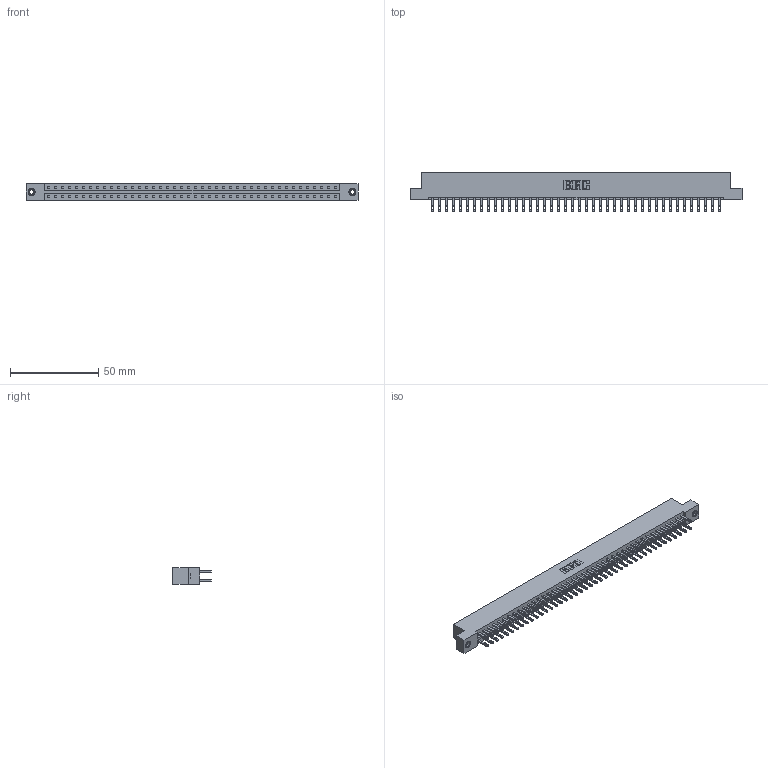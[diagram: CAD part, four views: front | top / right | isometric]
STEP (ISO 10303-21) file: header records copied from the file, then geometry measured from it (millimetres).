
FILE_DESCRIPTION (( 'STEP AP203' ), '1' );
FILE_NAME ('333-084-500-207.STEP', '2018-08-05T03:57:02', ( '' ), ( '' ), 'SwSTEP 2.0', 'SolidWorks 2016', '' );
FILE_SCHEMA (( 'CONFIG_CONTROL_DESIGN' ));
Length unit declared in the file: inch
Products named in the file (4): 333 Part_Flush - .156 Dia - TI; 345-292-001_345-293-100; 345-250-001_345-250-005-103; 333-084-500-207
Assembly tree (87 placements, depth 2):
  333-084-500-207
    333 Part_Flush - .156 Dia - TI
    345-292-001_345-293-100  x84
    345-250-001_345-250-005-103  x2
Bounding box: 187.96 x 21.85 x 9.4 mm (x, y, z)
Volume: 19432.8 mm3; surface area: 23932.9 mm2
Topology: 87 solids, 87 shells, 4206 faces, 12795 edges, 8522 vertices
Faces by surface type: plane 2622, cylinder 1568, cone 12, torus 4
Entity records: 28136 total; most frequent: CARTESIAN_POINT 4645, ORIENTED_EDGE 4574, DIRECTION 4001, EDGE_CURVE 2287, LINE 2135, VECTOR 2135, VERTEX_POINT 1520, AXIS2_PLACEMENT_3D 933
